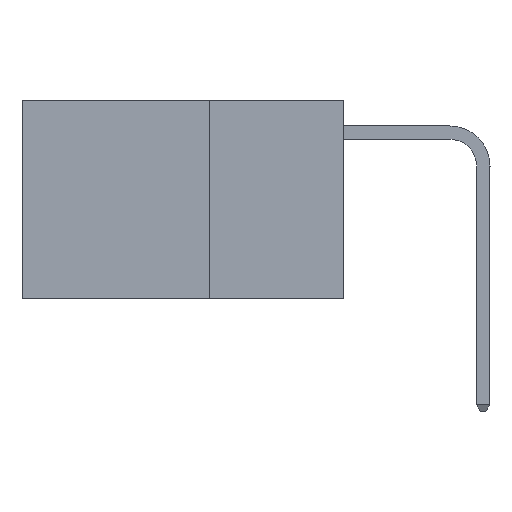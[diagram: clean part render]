
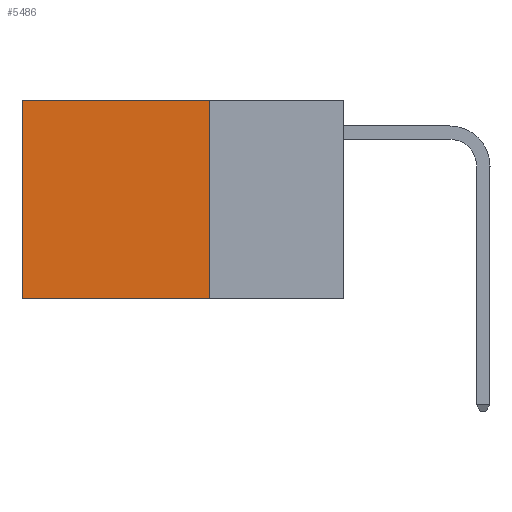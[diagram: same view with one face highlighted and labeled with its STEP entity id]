
A CAD part, left-side view. The second image highlights one B-rep face of the part: STEP entity #5486.
In plain terms, the highlighted planar face has unit normal (-1, 0, 0).
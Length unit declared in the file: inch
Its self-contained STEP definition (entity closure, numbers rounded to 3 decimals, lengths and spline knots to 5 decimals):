
#66 = VECTOR ( 'NONE', #93, 39.37008 ) ;
#93 = DIRECTION ( 'NONE',  ( 0., 0., -1. ) ) ;
#194 = VERTEX_POINT ( 'NONE', #5283 ) ;
#462 = ORIENTED_EDGE ( 'NONE', *, *, #4806, .F. ) ;
#786 = VERTEX_POINT ( 'NONE', #6226 ) ;
#2391 = PLANE ( 'NONE',  #6211 ) ;
#2690 = VECTOR ( 'NONE', #10617, 39.37008 ) ;
#3223 = CARTESIAN_POINT ( 'NONE',  ( 0.2625, 0.25, 0. ) ) ;
#3385 = CARTESIAN_POINT ( 'NONE',  ( 0.2625, 0.25, -0.37 ) ) ;
#3432 = VERTEX_POINT ( 'NONE', #8580 ) ;
#3470 = DIRECTION ( 'NONE',  ( 0., 0., -1. ) ) ;
#4455 = DIRECTION ( 'NONE',  ( 0., 1., 0. ) ) ;
#4493 = LINE ( 'NONE', #7695, #12530 ) ;
#4806 = EDGE_CURVE ( 'NONE', #6711, #3432, #13501, .T. ) ;
#5283 = CARTESIAN_POINT ( 'NONE',  ( 0.2625, 0.6, 0. ) ) ;
#5455 = EDGE_CURVE ( 'NONE', #786, #6711, #5846, .T. ) ;
#5486 = ADVANCED_FACE ( 'NONE', ( #13503 ), #2391, .F. ) ;
#5674 = CARTESIAN_POINT ( 'NONE',  ( 0.2625, 0.25, -0.37 ) ) ;
#5846 = LINE ( 'NONE', #9710, #66 ) ;
#5972 = EDGE_CURVE ( 'NONE', #194, #3432, #4493, .T. ) ;
#6152 = ORIENTED_EDGE ( 'NONE', *, *, #5455, .F. ) ;
#6211 = AXIS2_PLACEMENT_3D ( 'NONE', #6644, #9811, #3470 ) ;
#6226 = CARTESIAN_POINT ( 'NONE',  ( 0.2625, 0.25, 0. ) ) ;
#6644 = CARTESIAN_POINT ( 'NONE',  ( 0.2625, 0.25, 0. ) ) ;
#6711 = VERTEX_POINT ( 'NONE', #5674 ) ;
#7695 = CARTESIAN_POINT ( 'NONE',  ( 0.2625, 0.6, 0. ) ) ;
#8580 = CARTESIAN_POINT ( 'NONE',  ( 0.2625, 0.6, -0.37 ) ) ;
#8708 = DIRECTION ( 'NONE',  ( 0., 0., -1. ) ) ;
#8806 = ORIENTED_EDGE ( 'NONE', *, *, #5972, .T. ) ;
#9710 = CARTESIAN_POINT ( 'NONE',  ( 0.2625, 0.25, 0. ) ) ;
#9811 = DIRECTION ( 'NONE',  ( 1., 0., 0. ) ) ;
#10617 = DIRECTION ( 'NONE',  ( 0., 1., 0. ) ) ;
#10732 = EDGE_CURVE ( 'NONE', #786, #194, #13520, .T. ) ;
#12085 = VECTOR ( 'NONE', #4455, 39.37008 ) ;
#12530 = VECTOR ( 'NONE', #8708, 39.37008 ) ;
#12758 = ORIENTED_EDGE ( 'NONE', *, *, #10732, .T. ) ;
#13501 = LINE ( 'NONE', #3385, #12085 ) ;
#13503 = FACE_OUTER_BOUND ( 'NONE', #13663, .T. ) ;
#13520 = LINE ( 'NONE', #3223, #2690 ) ;
#13663 = EDGE_LOOP ( 'NONE', ( #8806, #462, #6152, #12758 ) ) ;
